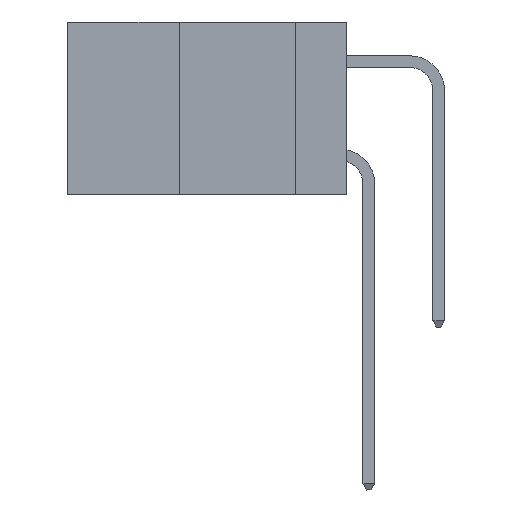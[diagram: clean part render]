
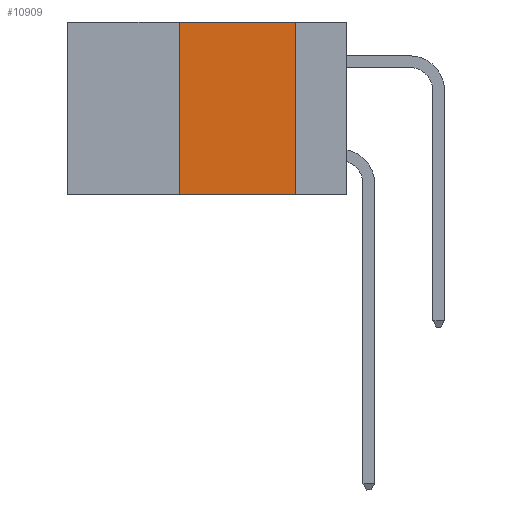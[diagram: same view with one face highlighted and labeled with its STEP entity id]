
A CAD part, left-side view. The second image highlights one B-rep face of the part: STEP entity #10909.
In plain terms, the highlighted planar face has unit normal (-1, 0, 0).
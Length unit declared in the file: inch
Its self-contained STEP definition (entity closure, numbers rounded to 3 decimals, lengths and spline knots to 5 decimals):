
#147 = VECTOR ( 'NONE', #3750, 39.37008 ) ;
#246 = DIRECTION ( 'NONE',  ( 1., 0., 0. ) ) ;
#453 = EDGE_CURVE ( 'NONE', #18332, #3034, #7807, .T. ) ;
#457 = AXIS2_PLACEMENT_3D ( 'NONE', #14434, #246, #12764 ) ;
#3034 = VERTEX_POINT ( 'NONE', #22262 ) ;
#3750 = DIRECTION ( 'NONE',  ( 0., -1., 0. ) ) ;
#4924 = CARTESIAN_POINT ( 'NONE',  ( 0., 0.36, 0. ) ) ;
#5014 = DIRECTION ( 'NONE',  ( 0., 0., -1. ) ) ;
#5867 = ORIENTED_EDGE ( 'NONE', *, *, #22884, .F. ) ;
#6220 = CARTESIAN_POINT ( 'NONE',  ( 0., 0.6, -0.37 ) ) ;
#6233 = FACE_OUTER_BOUND ( 'NONE', #9346, .T. ) ;
#6474 = ORIENTED_EDGE ( 'NONE', *, *, #453, .F. ) ;
#7244 = VECTOR ( 'NONE', #5014, 39.37008 ) ;
#7368 = PLANE ( 'NONE',  #457 ) ;
#7400 = ORIENTED_EDGE ( 'NONE', *, *, #12984, .F. ) ;
#7716 = CARTESIAN_POINT ( 'NONE',  ( 0., 0.11, 0. ) ) ;
#7807 = LINE ( 'NONE', #13040, #7244 ) ;
#8978 = ORIENTED_EDGE ( 'NONE', *, *, #12583, .T. ) ;
#9346 = EDGE_LOOP ( 'NONE', ( #6474, #7400, #5867, #8978 ) ) ;
#10229 = LINE ( 'NONE', #14447, #147 ) ;
#10673 = VERTEX_POINT ( 'NONE', #4924 ) ;
#10909 = ADVANCED_FACE ( 'NONE', ( #6233 ), #7368, .F. ) ;
#11655 = LINE ( 'NONE', #22441, #16324 ) ;
#12583 = EDGE_CURVE ( 'NONE', #22054, #3034, #13830, .T. ) ;
#12764 = DIRECTION ( 'NONE',  ( 0., 0., -1. ) ) ;
#12984 = EDGE_CURVE ( 'NONE', #10673, #18332, #10229, .T. ) ;
#13040 = CARTESIAN_POINT ( 'NONE',  ( 0., 0.11, 0. ) ) ;
#13336 = DIRECTION ( 'NONE',  ( 0., -1., 0. ) ) ;
#13830 = LINE ( 'NONE', #6220, #22590 ) ;
#14434 = CARTESIAN_POINT ( 'NONE',  ( 0., 0.6, 0. ) ) ;
#14447 = CARTESIAN_POINT ( 'NONE',  ( 0., 0.6, 0. ) ) ;
#16324 = VECTOR ( 'NONE', #18961, 39.37008 ) ;
#18332 = VERTEX_POINT ( 'NONE', #7716 ) ;
#18961 = DIRECTION ( 'NONE',  ( 0., 0., 1. ) ) ;
#21787 = CARTESIAN_POINT ( 'NONE',  ( 0., 0.36, -0.37 ) ) ;
#22054 = VERTEX_POINT ( 'NONE', #21787 ) ;
#22262 = CARTESIAN_POINT ( 'NONE',  ( 0., 0.11, -0.37 ) ) ;
#22441 = CARTESIAN_POINT ( 'NONE',  ( 0., 0.36, 0. ) ) ;
#22590 = VECTOR ( 'NONE', #13336, 39.37008 ) ;
#22884 = EDGE_CURVE ( 'NONE', #22054, #10673, #11655, .T. ) ;
